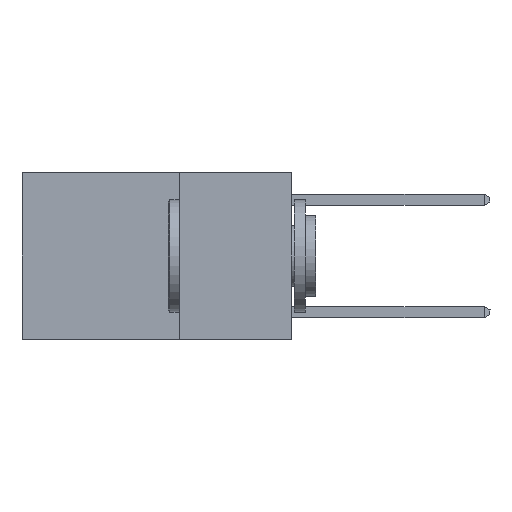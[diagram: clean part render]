
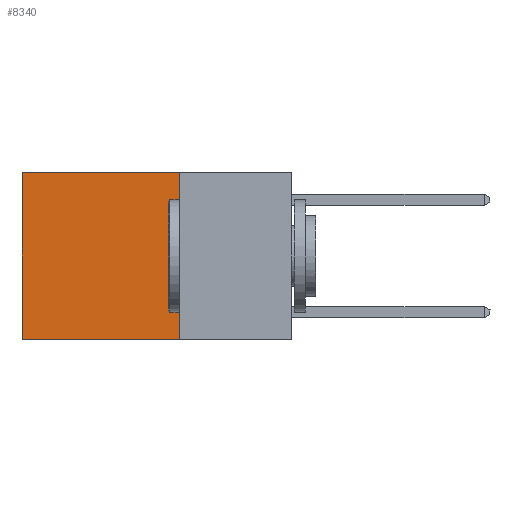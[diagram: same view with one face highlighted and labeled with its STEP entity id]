
A CAD part, left-side view. The second image highlights one B-rep face of the part: STEP entity #8340.
In plain terms, the highlighted planar face has unit normal (-1, 0, 0).
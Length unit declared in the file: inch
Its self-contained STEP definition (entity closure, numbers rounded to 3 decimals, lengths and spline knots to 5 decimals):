
#80 = EDGE_LOOP ( 'NONE', ( #16293, #5182, #13508, #12578 ) ) ;
#239 = DIRECTION ( 'NONE',  ( 0., 1., 0. ) ) ;
#1238 = CARTESIAN_POINT ( 'NONE',  ( 0.2625, 0.25, 0. ) ) ;
#1387 = EDGE_CURVE ( 'NONE', #20044, #6658, #4481, .T. ) ;
#2047 = EDGE_CURVE ( 'NONE', #6658, #8376, #12209, .T. ) ;
#2063 = LINE ( 'NONE', #11695, #24307 ) ;
#3324 = CARTESIAN_POINT ( 'NONE',  ( 0.2625, 0.6, 0. ) ) ;
#4030 = DIRECTION ( 'NONE',  ( 0., 0., -1. ) ) ;
#4481 = LINE ( 'NONE', #13005, #27175 ) ;
#5182 = ORIENTED_EDGE ( 'NONE', *, *, #2047, .F. ) ;
#5336 = EDGE_CURVE ( 'NONE', #20044, #10855, #2063, .T. ) ;
#5869 = CARTESIAN_POINT ( 'NONE',  ( 0.2625, 0.6, 0. ) ) ;
#6148 = LINE ( 'NONE', #3324, #17985 ) ;
#6658 = VERTEX_POINT ( 'NONE', #13424 ) ;
#8340 = ADVANCED_FACE ( 'NONE', ( #8712 ), #12499, .F. ) ;
#8376 = VERTEX_POINT ( 'NONE', #25818 ) ;
#8712 = FACE_OUTER_BOUND ( 'NONE', #80, .T. ) ;
#10294 = CARTESIAN_POINT ( 'NONE',  ( 0.2625, 0.25, 0. ) ) ;
#10855 = VERTEX_POINT ( 'NONE', #5869 ) ;
#11695 = CARTESIAN_POINT ( 'NONE',  ( 0.2625, 0.25, 0. ) ) ;
#12209 = LINE ( 'NONE', #21224, #23133 ) ;
#12499 = PLANE ( 'NONE',  #24980 ) ;
#12578 = ORIENTED_EDGE ( 'NONE', *, *, #5336, .T. ) ;
#12683 = DIRECTION ( 'NONE',  ( 1., 0., 0. ) ) ;
#13005 = CARTESIAN_POINT ( 'NONE',  ( 0.2625, 0.25, 0. ) ) ;
#13424 = CARTESIAN_POINT ( 'NONE',  ( 0.2625, 0.25, -0.37 ) ) ;
#13508 = ORIENTED_EDGE ( 'NONE', *, *, #1387, .F. ) ;
#16293 = ORIENTED_EDGE ( 'NONE', *, *, #16729, .T. ) ;
#16729 = EDGE_CURVE ( 'NONE', #10855, #8376, #6148, .T. ) ;
#17985 = VECTOR ( 'NONE', #18956, 39.37008 ) ;
#18956 = DIRECTION ( 'NONE',  ( 0., 0., -1. ) ) ;
#20044 = VERTEX_POINT ( 'NONE', #10294 ) ;
#21224 = CARTESIAN_POINT ( 'NONE',  ( 0.2625, 0.25, -0.37 ) ) ;
#23133 = VECTOR ( 'NONE', #27669, 39.37008 ) ;
#24307 = VECTOR ( 'NONE', #239, 39.37008 ) ;
#24980 = AXIS2_PLACEMENT_3D ( 'NONE', #1238, #12683, #27820 ) ;
#25818 = CARTESIAN_POINT ( 'NONE',  ( 0.2625, 0.6, -0.37 ) ) ;
#27175 = VECTOR ( 'NONE', #4030, 39.37008 ) ;
#27669 = DIRECTION ( 'NONE',  ( 0., 1., 0. ) ) ;
#27820 = DIRECTION ( 'NONE',  ( 0., 0., -1. ) ) ;
